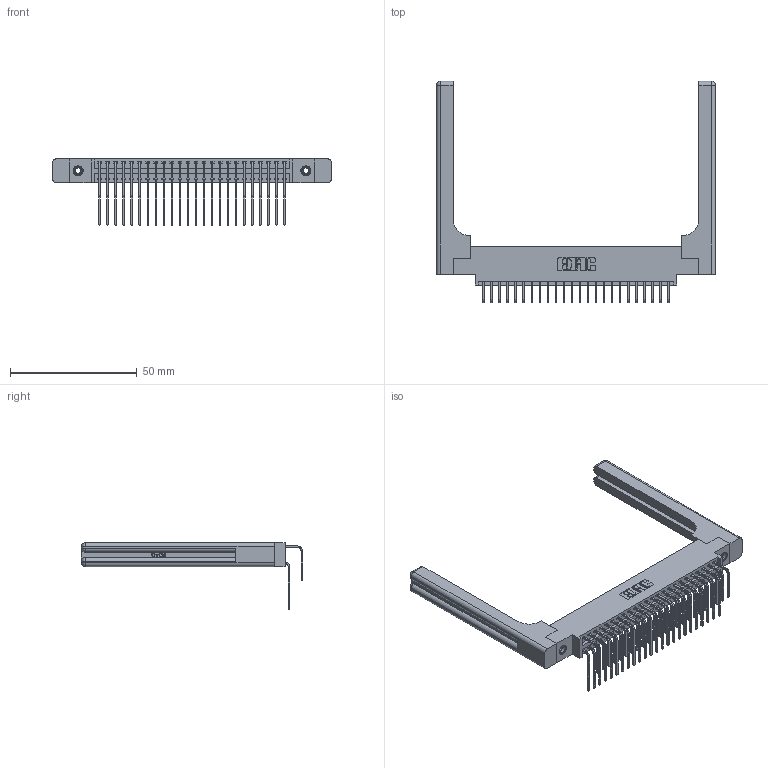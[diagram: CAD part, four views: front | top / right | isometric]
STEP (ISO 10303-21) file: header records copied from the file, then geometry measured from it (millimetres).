
FILE_DESCRIPTION (( 'STEP AP203' ), '1' );
FILE_NAME ('346-048-558-858.STEP', '2022-05-20T22:11:20', ( '' ), ( '' ), 'SwSTEP 2.0', 'SolidWorks 2020', '' );
FILE_SCHEMA (( 'CONFIG_CONTROL_DESIGN' ));
Length unit declared in the file: inch
Products named in the file (6): 346-220-058_345-220-058; 345-292-001_558 Tail - 2; 345-250-001_345-250-001-102; 345-292-001_558 559 Tail - 1; 346 Part_0.170 Offset - 0.156 Dia-TH; 346-048-558-858
Assembly tree (53 placements, depth 2):
  346-048-558-858
    346 Part_0.170 Offset - 0.156 Dia-TH
    345-292-001_558 559 Tail - 1  x24
    345-292-001_558 Tail - 2  x24
    345-250-001_345-250-001-102  x2
    346-220-058_345-220-058  x2
Bounding box: 110.26 x 87.44 x 26.16 mm (x, y, z)
Volume: 18210.5 mm3; surface area: 20962.6 mm2
Topology: 53 solids, 53 shells, 2988 faces, 8771 edges, 5762 vertices
Faces by surface type: plane 2018, cylinder 910, bspline 36, cone 12, sphere 8, torus 4
Entity records: 25600 total; most frequent: CARTESIAN_POINT 5310, ORIENTED_EDGE 3988, DIRECTION 3634, EDGE_CURVE 1994, LINE 1634, VECTOR 1634, VERTEX_POINT 1318, AXIS2_PLACEMENT_3D 1000
